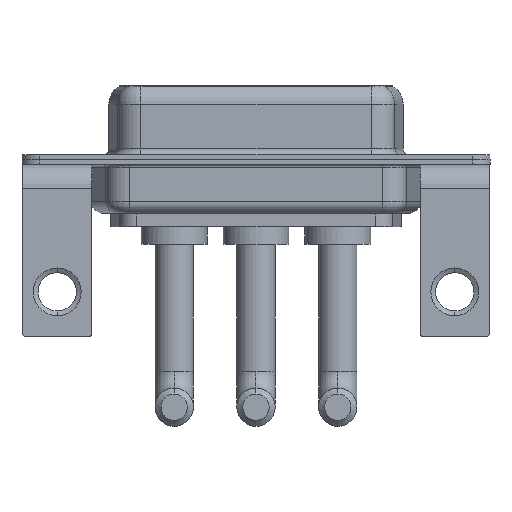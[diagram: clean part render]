
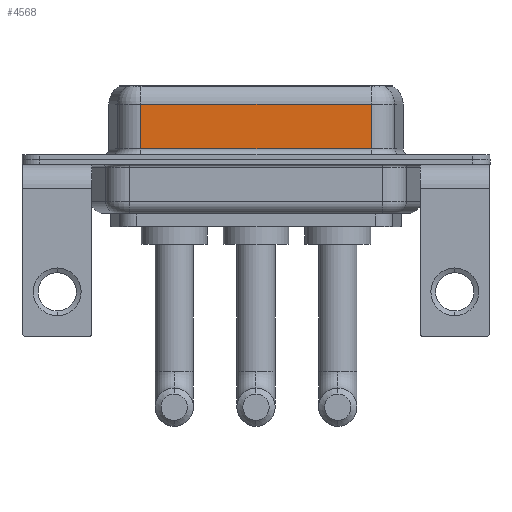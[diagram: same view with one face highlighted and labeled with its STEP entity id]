
A CAD part, front view. The second image highlights one B-rep face of the part: STEP entity #4568.
In plain terms, the highlighted planar face has unit normal (0, -1, 0).
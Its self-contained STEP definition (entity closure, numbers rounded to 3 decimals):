
#338 = ORIENTED_EDGE ( 'NONE', *, *, #2728, .T. ) ;
#1202 = ORIENTED_EDGE ( 'NONE', *, *, #8015, .T. ) ;
#1683 = CARTESIAN_POINT ( 'NONE',  ( 26.287, -3.95, 0.9 ) ) ;
#1895 = CARTESIAN_POINT ( 'NONE',  ( 7.013, -3.95, 6.4 ) ) ;
#2294 = ORIENTED_EDGE ( 'NONE', *, *, #7724, .F. ) ;
#2721 = DIRECTION ( 'NONE',  ( 0., 1., 0. ) ) ;
#2728 = EDGE_CURVE ( 'NONE', #6400, #11719, #4151, .T. ) ;
#4151 = LINE ( 'NONE', #1895, #9349 ) ;
#4437 = VECTOR ( 'NONE', #6775, 1000. ) ;
#4568 = ADVANCED_FACE ( 'NONE', ( #8591 ), #5772, .F. ) ;
#4792 = CARTESIAN_POINT ( 'NONE',  ( 26.287, -3.95, 4.65 ) ) ;
#5052 = VECTOR ( 'NONE', #12528, 1000. ) ;
#5672 = CARTESIAN_POINT ( 'NONE',  ( 26.287, -3.95, 4.65 ) ) ;
#5692 = VECTOR ( 'NONE', #13004, 1000. ) ;
#5772 = PLANE ( 'NONE',  #10259 ) ;
#5982 = CARTESIAN_POINT ( 'NONE',  ( 7.013, -3.95, 0.9 ) ) ;
#6400 = VERTEX_POINT ( 'NONE', #8051 ) ;
#6626 = EDGE_CURVE ( 'NONE', #11719, #10759, #8504, .T. ) ;
#6775 = DIRECTION ( 'NONE',  ( -1., 0., 0. ) ) ;
#7396 = ORIENTED_EDGE ( 'NONE', *, *, #6626, .T. ) ;
#7636 = CARTESIAN_POINT ( 'NONE',  ( 26.287, -3.95, 0.9 ) ) ;
#7724 = EDGE_CURVE ( 'NONE', #8994, #10759, #11031, .T. ) ;
#8015 = EDGE_CURVE ( 'NONE', #8994, #6400, #10805, .T. ) ;
#8051 = CARTESIAN_POINT ( 'NONE',  ( 7.013, -3.95, 4.65 ) ) ;
#8504 = LINE ( 'NONE', #7636, #5052 ) ;
#8591 = FACE_OUTER_BOUND ( 'NONE', #9588, .T. ) ;
#8790 = DIRECTION ( 'NONE',  ( 0., 0., 1. ) ) ;
#8994 = VERTEX_POINT ( 'NONE', #4792 ) ;
#9036 = DIRECTION ( 'NONE',  ( 0., 0., -1. ) ) ;
#9349 = VECTOR ( 'NONE', #9036, 1000. ) ;
#9588 = EDGE_LOOP ( 'NONE', ( #2294, #1202, #338, #7396 ) ) ;
#10173 = CARTESIAN_POINT ( 'NONE',  ( 26.287, -3.95, 6.4 ) ) ;
#10259 = AXIS2_PLACEMENT_3D ( 'NONE', #10762, #2721, #8790 ) ;
#10759 = VERTEX_POINT ( 'NONE', #1683 ) ;
#10762 = CARTESIAN_POINT ( 'NONE',  ( 26.287, -3.95, 6.4 ) ) ;
#10805 = LINE ( 'NONE', #5672, #4437 ) ;
#11031 = LINE ( 'NONE', #10173, #5692 ) ;
#11719 = VERTEX_POINT ( 'NONE', #5982 ) ;
#12528 = DIRECTION ( 'NONE',  ( 1., 0., 0. ) ) ;
#13004 = DIRECTION ( 'NONE',  ( 0., 0., -1. ) ) ;
